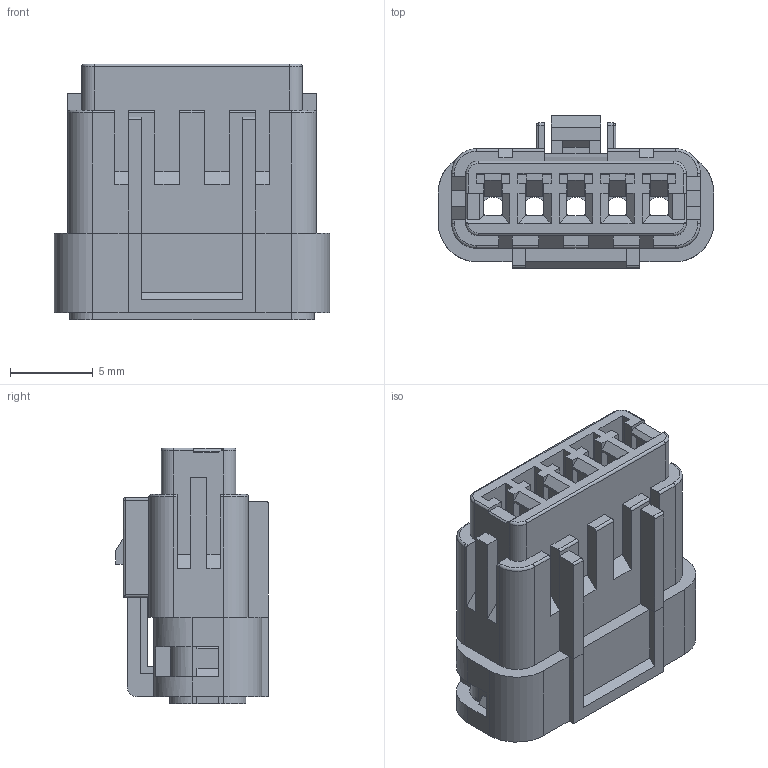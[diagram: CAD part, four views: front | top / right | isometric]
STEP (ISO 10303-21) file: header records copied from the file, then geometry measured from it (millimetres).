
FILE_DESCRIPTION (( 'STEP AP214' ), '1' );
FILE_NAME ('565-005-000-411.STEP', '2020-07-27T16:00:27', ( '' ), ( '' ), 'SwSTEP 2.0', 'SolidWorks 2020', '' );
FILE_SCHEMA (( 'AUTOMOTIVE_DESIGN' ));
Length unit declared in the file: millimetre
Products named in the file (4): 565-005-000-411_Rear Insulator; 565-005-000-411; 565-005-000-411_Rear Gasket; 565-005-000-411_Housing
Assembly tree (3 placements, depth 2):
  565-005-000-411
    565-005-000-411_Housing
    565-005-000-411_Rear Insulator
    565-005-000-411_Rear Gasket
Bounding box: 16.6 x 9.2 x 15.44 mm (x, y, z)
Volume: 979.9 mm3; surface area: 2530.8 mm2
Topology: 7 solids, 7 shells, 483 faces, 1344 edges, 881 vertices
Faces by surface type: plane 356, cylinder 99, torus 18, bspline 8, sphere 2
Entity records: 15967 total; most frequent: CARTESIAN_POINT 3196, ORIENTED_EDGE 2684, DIRECTION 2521, EDGE_CURVE 1342, LINE 1085, VECTOR 1085, VERTEX_POINT 881, AXIS2_PLACEMENT_3D 718
